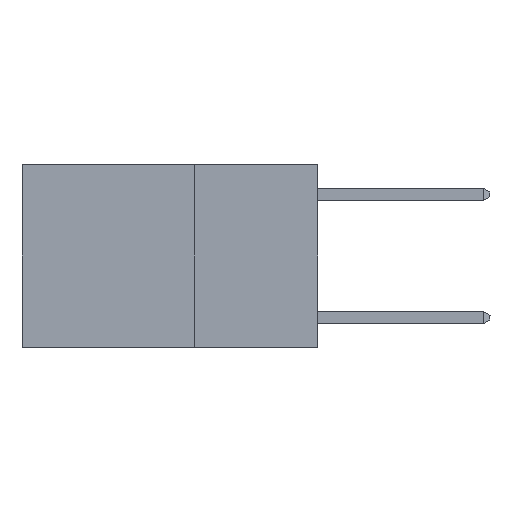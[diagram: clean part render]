
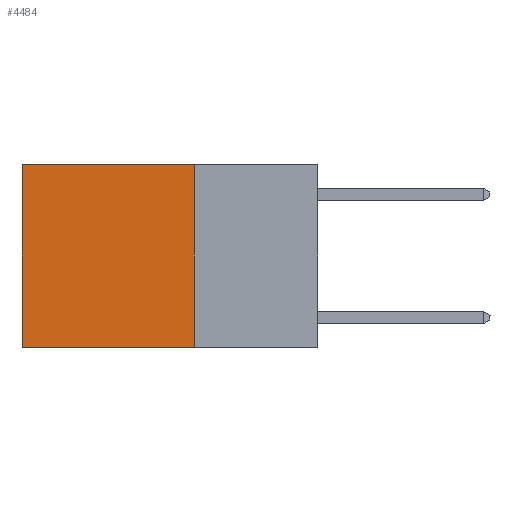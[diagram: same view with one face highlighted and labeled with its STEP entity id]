
A CAD part, left-side view. The second image highlights one B-rep face of the part: STEP entity #4484.
In plain terms, the highlighted planar face has unit normal (-1, 0, 0).
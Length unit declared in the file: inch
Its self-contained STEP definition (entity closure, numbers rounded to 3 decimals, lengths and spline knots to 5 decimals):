
#238 = CARTESIAN_POINT ( 'NONE',  ( 0.2625, 0.25, 0. ) ) ;
#287 = VERTEX_POINT ( 'NONE', #1049 ) ;
#317 = VERTEX_POINT ( 'NONE', #376 ) ;
#350 = AXIS2_PLACEMENT_3D ( 'NONE', #1892, #2783, #8366 ) ;
#376 = CARTESIAN_POINT ( 'NONE',  ( 0.2625, 0.25, -0.37 ) ) ;
#965 = PLANE ( 'NONE',  #350 ) ;
#993 = EDGE_CURVE ( 'NONE', #317, #287, #2488, .T. ) ;
#1049 = CARTESIAN_POINT ( 'NONE',  ( 0.2625, 0.6, -0.37 ) ) ;
#1350 = VERTEX_POINT ( 'NONE', #10088 ) ;
#1629 = VECTOR ( 'NONE', #5273, 39.37008 ) ;
#1892 = CARTESIAN_POINT ( 'NONE',  ( 0.2625, 0.25, 0. ) ) ;
#2255 = ORIENTED_EDGE ( 'NONE', *, *, #9180, .F. ) ;
#2358 = EDGE_CURVE ( 'NONE', #8035, #287, #3908, .T. ) ;
#2488 = LINE ( 'NONE', #5970, #6844 ) ;
#2783 = DIRECTION ( 'NONE',  ( 1., 0., 0. ) ) ;
#2910 = DIRECTION ( 'NONE',  ( 0., 1., 0. ) ) ;
#3578 = ORIENTED_EDGE ( 'NONE', *, *, #2358, .T. ) ;
#3889 = FACE_OUTER_BOUND ( 'NONE', #5389, .T. ) ;
#3908 = LINE ( 'NONE', #9089, #1629 ) ;
#4076 = DIRECTION ( 'NONE',  ( 0., 0., -1. ) ) ;
#4484 = ADVANCED_FACE ( 'NONE', ( #3889 ), #965, .F. ) ;
#4893 = CARTESIAN_POINT ( 'NONE',  ( 0.2625, 0.6, 0. ) ) ;
#4966 = VECTOR ( 'NONE', #4076, 39.37008 ) ;
#5148 = ORIENTED_EDGE ( 'NONE', *, *, #7197, .T. ) ;
#5273 = DIRECTION ( 'NONE',  ( 0., 0., -1. ) ) ;
#5389 = EDGE_LOOP ( 'NONE', ( #3578, #9568, #2255, #5148 ) ) ;
#5658 = LINE ( 'NONE', #238, #7475 ) ;
#5970 = CARTESIAN_POINT ( 'NONE',  ( 0.2625, 0.25, -0.37 ) ) ;
#6542 = CARTESIAN_POINT ( 'NONE',  ( 0.2625, 0.25, 0. ) ) ;
#6844 = VECTOR ( 'NONE', #9716, 39.37008 ) ;
#7197 = EDGE_CURVE ( 'NONE', #1350, #8035, #5658, .T. ) ;
#7475 = VECTOR ( 'NONE', #2910, 39.37008 ) ;
#8035 = VERTEX_POINT ( 'NONE', #4893 ) ;
#8366 = DIRECTION ( 'NONE',  ( 0., 0., -1. ) ) ;
#9063 = LINE ( 'NONE', #6542, #4966 ) ;
#9089 = CARTESIAN_POINT ( 'NONE',  ( 0.2625, 0.6, 0. ) ) ;
#9180 = EDGE_CURVE ( 'NONE', #1350, #317, #9063, .T. ) ;
#9568 = ORIENTED_EDGE ( 'NONE', *, *, #993, .F. ) ;
#9716 = DIRECTION ( 'NONE',  ( 0., 1., 0. ) ) ;
#10088 = CARTESIAN_POINT ( 'NONE',  ( 0.2625, 0.25, 0. ) ) ;
